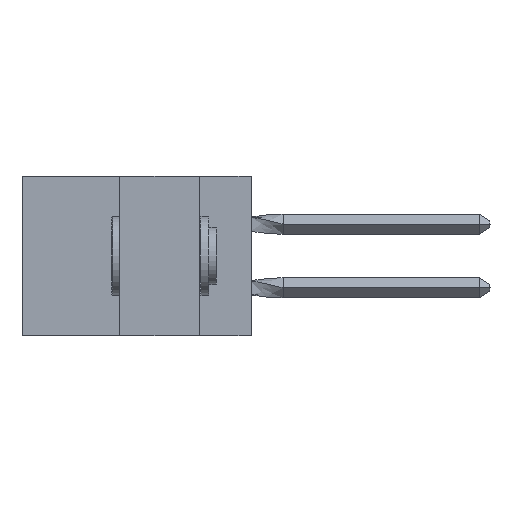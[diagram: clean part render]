
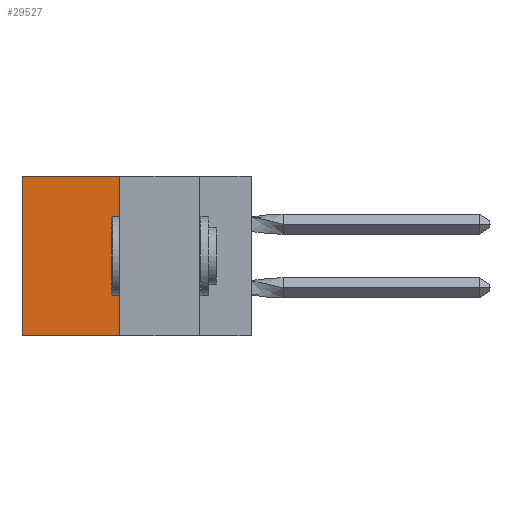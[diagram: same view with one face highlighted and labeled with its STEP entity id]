
A CAD part, left-side view. The second image highlights one B-rep face of the part: STEP entity #29527.
In plain terms, the highlighted planar face has unit normal (-1, 0, 0).
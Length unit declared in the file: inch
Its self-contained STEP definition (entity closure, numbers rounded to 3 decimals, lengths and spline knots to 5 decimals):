
#204 = CARTESIAN_POINT ( 'NONE',  ( 0.305, 0.413, -0.5 ) ) ;
#680 = DIRECTION ( 'NONE',  ( 0., 0., -1. ) ) ;
#893 = LINE ( 'NONE', #28880, #32538 ) ;
#1385 = LINE ( 'NONE', #1936, #30299 ) ;
#1436 = VECTOR ( 'NONE', #7941, 39.37008 ) ;
#1936 = CARTESIAN_POINT ( 'NONE',  ( 0.305, 0.413, -0.5 ) ) ;
#2005 = VERTEX_POINT ( 'NONE', #9170 ) ;
#2924 = PLANE ( 'NONE',  #34459 ) ;
#3753 = EDGE_CURVE ( 'NONE', #28536, #10352, #16314, .T. ) ;
#5082 = CARTESIAN_POINT ( 'NONE',  ( 0.305, 0.72, -0.5 ) ) ;
#7897 = VECTOR ( 'NONE', #12730, 39.37008 ) ;
#7941 = DIRECTION ( 'NONE',  ( 0., 0., -1. ) ) ;
#8206 = ORIENTED_EDGE ( 'NONE', *, *, #13977, .F. ) ;
#8910 = DIRECTION ( 'NONE',  ( 0., 0., -1. ) ) ;
#8991 = LINE ( 'NONE', #5082, #1436 ) ;
#9170 = CARTESIAN_POINT ( 'NONE',  ( 0.305, 0.72, -0.5 ) ) ;
#9270 = CARTESIAN_POINT ( 'NONE',  ( 0.305, 0.413, -0.5 ) ) ;
#10352 = VERTEX_POINT ( 'NONE', #35323 ) ;
#10641 = CARTESIAN_POINT ( 'NONE',  ( 0.305, 0.413, 0. ) ) ;
#11792 = EDGE_LOOP ( 'NONE', ( #34251, #20071, #8206, #14172 ) ) ;
#12627 = EDGE_CURVE ( 'NONE', #30226, #2005, #1385, .T. ) ;
#12730 = DIRECTION ( 'NONE',  ( 0., 1., 0. ) ) ;
#13977 = EDGE_CURVE ( 'NONE', #28536, #30226, #893, .T. ) ;
#14172 = ORIENTED_EDGE ( 'NONE', *, *, #3753, .T. ) ;
#14484 = DIRECTION ( 'NONE',  ( 1., 0., 0. ) ) ;
#16314 = LINE ( 'NONE', #21269, #7897 ) ;
#20071 = ORIENTED_EDGE ( 'NONE', *, *, #12627, .F. ) ;
#21269 = CARTESIAN_POINT ( 'NONE',  ( 0.305, 0.413, 0. ) ) ;
#21792 = DIRECTION ( 'NONE',  ( 0., 1., 0. ) ) ;
#24166 = EDGE_CURVE ( 'NONE', #10352, #2005, #8991, .T. ) ;
#28041 = FACE_OUTER_BOUND ( 'NONE', #11792, .T. ) ;
#28536 = VERTEX_POINT ( 'NONE', #10641 ) ;
#28880 = CARTESIAN_POINT ( 'NONE',  ( 0.305, 0.413, -0.5 ) ) ;
#29527 = ADVANCED_FACE ( 'NONE', ( #28041 ), #2924, .F. ) ;
#30226 = VERTEX_POINT ( 'NONE', #9270 ) ;
#30299 = VECTOR ( 'NONE', #21792, 39.37008 ) ;
#32538 = VECTOR ( 'NONE', #680, 39.37008 ) ;
#34251 = ORIENTED_EDGE ( 'NONE', *, *, #24166, .T. ) ;
#34459 = AXIS2_PLACEMENT_3D ( 'NONE', #204, #14484, #8910 ) ;
#35323 = CARTESIAN_POINT ( 'NONE',  ( 0.305, 0.72, 0. ) ) ;
